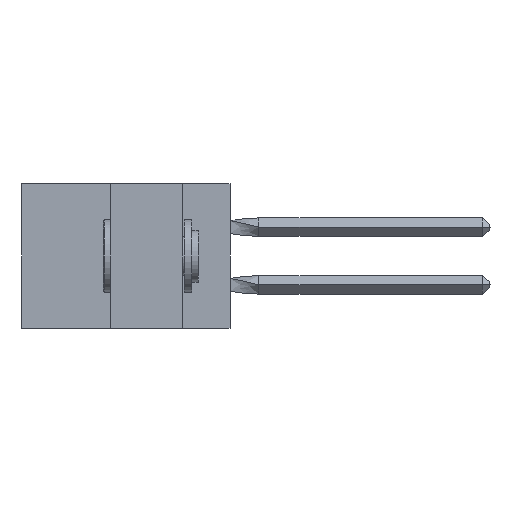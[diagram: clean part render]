
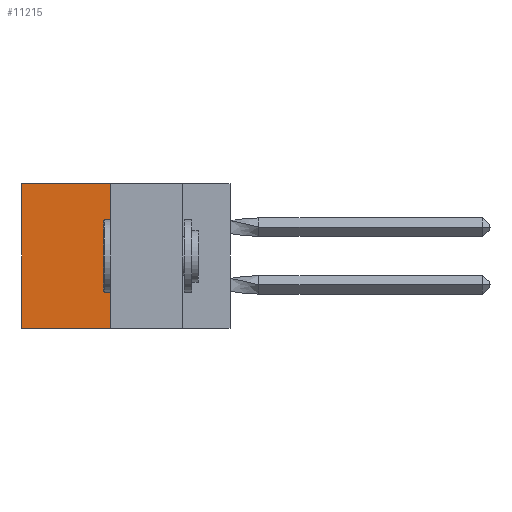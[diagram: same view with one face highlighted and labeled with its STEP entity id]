
A CAD part, left-side view. The second image highlights one B-rep face of the part: STEP entity #11215.
In plain terms, the highlighted planar face has unit normal (-1, 0, 0).
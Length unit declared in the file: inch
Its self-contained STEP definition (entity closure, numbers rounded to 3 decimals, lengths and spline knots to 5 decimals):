
#229 = FACE_OUTER_BOUND ( 'NONE', #23204, .T. ) ;
#1018 = VERTEX_POINT ( 'NONE', #32482 ) ;
#3550 = CARTESIAN_POINT ( 'NONE',  ( 0.305, 0.413, -0.5 ) ) ;
#3660 = LINE ( 'NONE', #7709, #18227 ) ;
#6082 = VECTOR ( 'NONE', #15479, 39.37008 ) ;
#7345 = DIRECTION ( 'NONE',  ( 0., 0., -1. ) ) ;
#7709 = CARTESIAN_POINT ( 'NONE',  ( 0.305, 0.413, -0.5 ) ) ;
#7934 = VERTEX_POINT ( 'NONE', #24804 ) ;
#9249 = VERTEX_POINT ( 'NONE', #35668 ) ;
#11215 = ADVANCED_FACE ( 'NONE', ( #229 ), #17186, .F. ) ;
#12699 = ORIENTED_EDGE ( 'NONE', *, *, #30853, .T. ) ;
#13387 = LINE ( 'NONE', #3550, #26092 ) ;
#15479 = DIRECTION ( 'NONE',  ( 0., 1., 0. ) ) ;
#17057 = CARTESIAN_POINT ( 'NONE',  ( 0.305, 0.413, -0.5 ) ) ;
#17186 = PLANE ( 'NONE',  #23817 ) ;
#18227 = VECTOR ( 'NONE', #7345, 39.37008 ) ;
#19982 = DIRECTION ( 'NONE',  ( 1., 0., 0. ) ) ;
#20325 = ORIENTED_EDGE ( 'NONE', *, *, #34971, .F. ) ;
#20421 = DIRECTION ( 'NONE',  ( 0., 1., 0. ) ) ;
#23175 = DIRECTION ( 'NONE',  ( 0., 0., -1. ) ) ;
#23204 = EDGE_LOOP ( 'NONE', ( #12699, #20325, #26470, #32964 ) ) ;
#23607 = EDGE_CURVE ( 'NONE', #7934, #37511, #32161, .T. ) ;
#23817 = AXIS2_PLACEMENT_3D ( 'NONE', #17057, #19982, #23175 ) ;
#24804 = CARTESIAN_POINT ( 'NONE',  ( 0.305, 0.413, 0. ) ) ;
#26092 = VECTOR ( 'NONE', #20421, 39.37008 ) ;
#26470 = ORIENTED_EDGE ( 'NONE', *, *, #35956, .F. ) ;
#30853 = EDGE_CURVE ( 'NONE', #37511, #9249, #34644, .T. ) ;
#31155 = CARTESIAN_POINT ( 'NONE',  ( 0.305, 0.72, -0.5 ) ) ;
#32161 = LINE ( 'NONE', #32607, #6082 ) ;
#32366 = VECTOR ( 'NONE', #36895, 39.37008 ) ;
#32482 = CARTESIAN_POINT ( 'NONE',  ( 0.305, 0.413, -0.5 ) ) ;
#32607 = CARTESIAN_POINT ( 'NONE',  ( 0.305, 0.413, 0. ) ) ;
#32964 = ORIENTED_EDGE ( 'NONE', *, *, #23607, .T. ) ;
#34644 = LINE ( 'NONE', #31155, #32366 ) ;
#34971 = EDGE_CURVE ( 'NONE', #1018, #9249, #13387, .T. ) ;
#35668 = CARTESIAN_POINT ( 'NONE',  ( 0.305, 0.72, -0.5 ) ) ;
#35956 = EDGE_CURVE ( 'NONE', #7934, #1018, #3660, .T. ) ;
#36895 = DIRECTION ( 'NONE',  ( 0., 0., -1. ) ) ;
#37511 = VERTEX_POINT ( 'NONE', #37750 ) ;
#37750 = CARTESIAN_POINT ( 'NONE',  ( 0.305, 0.72, 0. ) ) ;
